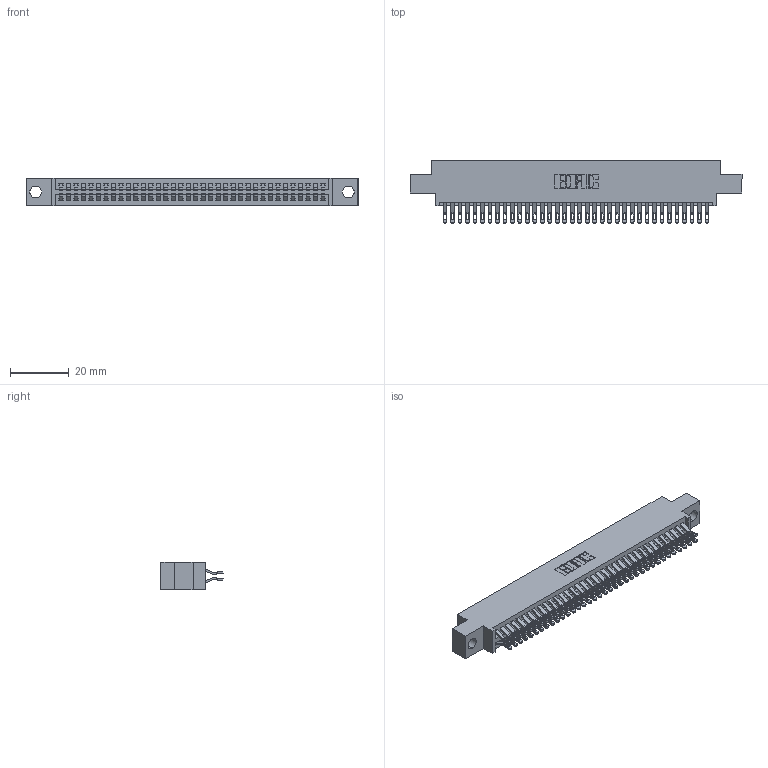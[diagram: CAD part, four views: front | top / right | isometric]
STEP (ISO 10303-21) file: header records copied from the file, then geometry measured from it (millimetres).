
FILE_DESCRIPTION (( 'STEP AP203' ), '1' );
FILE_NAME ('345-072-555-804.STEP', '2021-05-20T09:03:29', ( '' ), ( '' ), 'SwSTEP 2.0', 'SolidWorks 2020', '' );
FILE_SCHEMA (( 'CONFIG_CONTROL_DESIGN' ));
Length unit declared in the file: inch
Products named in the file (3): 345-292-001_555 Tail; 345 Part_0.170 Offset - 0.156 Dia-TI; 345-072-555-804
Assembly tree (73 placements, depth 2):
  345-072-555-804
    345 Part_0.170 Offset - 0.156 Dia-TI
    345-292-001_555 Tail  x72
Bounding box: 112.65 x 21.13 x 9.4 mm (x, y, z)
Volume: 10876.6 mm3; surface area: 16682.7 mm2
Topology: 73 solids, 73 shells, 4176 faces, 13133 edges, 8754 vertices
Faces by surface type: plane 2330, cylinder 1846
Entity records: 29931 total; most frequent: CARTESIAN_POINT 5064, ORIENTED_EDGE 4966, DIRECTION 4439, EDGE_CURVE 2483, VECTOR 2187, LINE 2187, VERTEX_POINT 1654, AXIS2_PLACEMENT_3D 1126
